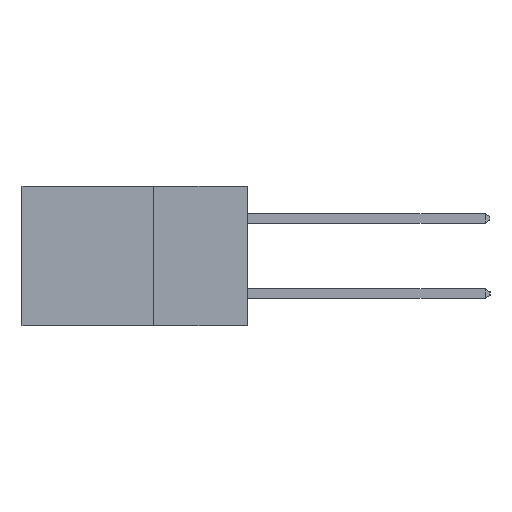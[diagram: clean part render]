
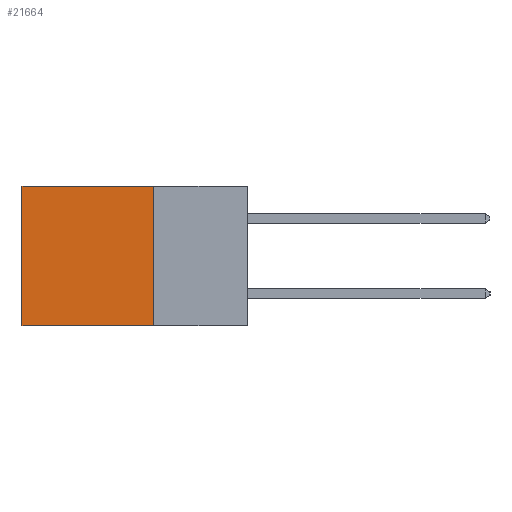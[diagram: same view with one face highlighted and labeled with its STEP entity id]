
A CAD part, left-side view. The second image highlights one B-rep face of the part: STEP entity #21664.
In plain terms, the highlighted planar face has unit normal (-1, 0, 0).
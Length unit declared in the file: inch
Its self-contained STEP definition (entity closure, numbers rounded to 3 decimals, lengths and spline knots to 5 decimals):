
#184 = PLANE ( 'NONE',  #26689 ) ;
#412 = EDGE_LOOP ( 'NONE', ( #9055, #9686, #14310, #10524 ) ) ;
#1419 = DIRECTION ( 'NONE',  ( 0., 0., -1. ) ) ;
#2993 = CARTESIAN_POINT ( 'NONE',  ( 0.2615, 0.25, 0. ) ) ;
#3199 = VECTOR ( 'NONE', #8198, 39.37008 ) ;
#4395 = DIRECTION ( 'NONE',  ( 1., 0., 0. ) ) ;
#5706 = VERTEX_POINT ( 'NONE', #20998 ) ;
#5910 = EDGE_CURVE ( 'NONE', #12770, #5706, #9572, .T. ) ;
#6079 = CARTESIAN_POINT ( 'NONE',  ( 0.2615, 0.25, -0.37 ) ) ;
#6807 = CARTESIAN_POINT ( 'NONE',  ( 0.2615, 0.25, -0.37 ) ) ;
#8198 = DIRECTION ( 'NONE',  ( 0., 0., -1. ) ) ;
#9055 = ORIENTED_EDGE ( 'NONE', *, *, #9566, .T. ) ;
#9212 = VECTOR ( 'NONE', #11077, 39.37008 ) ;
#9317 = DIRECTION ( 'NONE',  ( 0., 1., 0. ) ) ;
#9566 = EDGE_CURVE ( 'NONE', #5706, #17212, #21381, .T. ) ;
#9572 = LINE ( 'NONE', #2993, #14476 ) ;
#9686 = ORIENTED_EDGE ( 'NONE', *, *, #13740, .F. ) ;
#10524 = ORIENTED_EDGE ( 'NONE', *, *, #5910, .T. ) ;
#11077 = DIRECTION ( 'NONE',  ( 0., 1., 0. ) ) ;
#12770 = VERTEX_POINT ( 'NONE', #13252 ) ;
#13252 = CARTESIAN_POINT ( 'NONE',  ( 0.2615, 0.25, 0. ) ) ;
#13740 = EDGE_CURVE ( 'NONE', #23835, #17212, #20233, .T. ) ;
#14310 = ORIENTED_EDGE ( 'NONE', *, *, #15569, .F. ) ;
#14476 = VECTOR ( 'NONE', #9317, 39.37008 ) ;
#14818 = CARTESIAN_POINT ( 'NONE',  ( 0.2615, 0.6, -0.37 ) ) ;
#15569 = EDGE_CURVE ( 'NONE', #12770, #23835, #19791, .T. ) ;
#17212 = VERTEX_POINT ( 'NONE', #14818 ) ;
#18866 = CARTESIAN_POINT ( 'NONE',  ( 0.2615, 0.25, -0.37 ) ) ;
#18954 = DIRECTION ( 'NONE',  ( 0., 0., -1. ) ) ;
#19791 = LINE ( 'NONE', #6079, #3199 ) ;
#20158 = CARTESIAN_POINT ( 'NONE',  ( 0.2615, 0.6, -0.37 ) ) ;
#20233 = LINE ( 'NONE', #6807, #9212 ) ;
#20998 = CARTESIAN_POINT ( 'NONE',  ( 0.2615, 0.6, 0. ) ) ;
#21381 = LINE ( 'NONE', #20158, #26089 ) ;
#21664 = ADVANCED_FACE ( 'NONE', ( #26670 ), #184, .F. ) ;
#23361 = CARTESIAN_POINT ( 'NONE',  ( 0.2615, 0.25, -0.37 ) ) ;
#23835 = VERTEX_POINT ( 'NONE', #23361 ) ;
#26089 = VECTOR ( 'NONE', #1419, 39.37008 ) ;
#26670 = FACE_OUTER_BOUND ( 'NONE', #412, .T. ) ;
#26689 = AXIS2_PLACEMENT_3D ( 'NONE', #18866, #4395, #18954 ) ;
